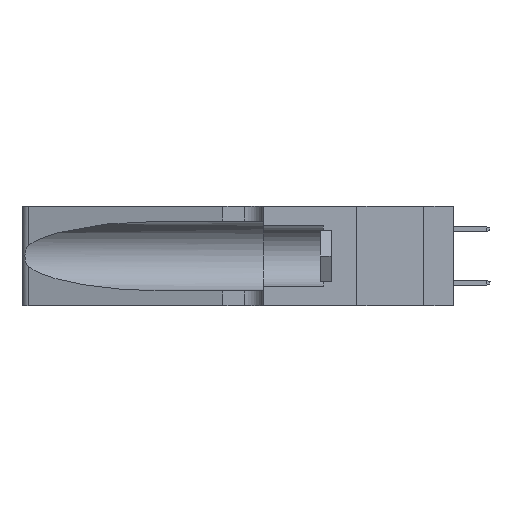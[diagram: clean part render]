
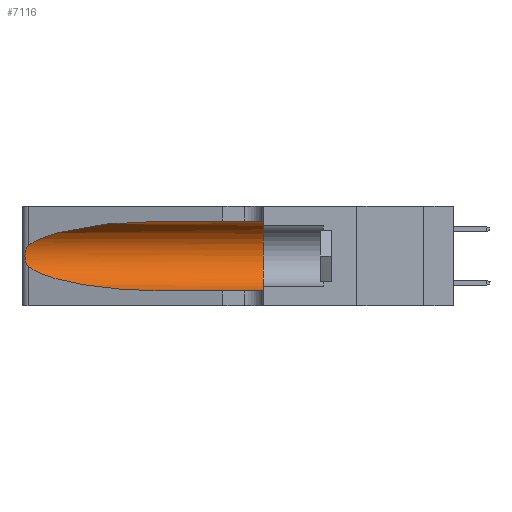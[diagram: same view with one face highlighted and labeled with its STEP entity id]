
A CAD part, left-side view. The second image highlights one B-rep face of the part: STEP entity #7116.
In plain terms, the highlighted cylindrical face has radius 3.308 mm (diameter 6.617 mm), a partial arc.
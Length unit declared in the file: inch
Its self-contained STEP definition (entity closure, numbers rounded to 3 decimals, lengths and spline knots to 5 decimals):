
#10 = CARTESIAN_POINT ( 'NONE',  ( 0.26075, 1.23896, 0.178 ) ) ;
#398 = CARTESIAN_POINT ( 'NONE',  ( 0.25487, 1.22718, 0.22369 ) ) ;
#905 = CARTESIAN_POINT ( 'NONE',  ( 0.18966, 0.96281, 0.31525 ) ) ;
#1256 = ORIENTED_EDGE ( 'NONE', *, *, #2125, .T. ) ;
#1506 = VERTEX_POINT ( 'NONE', #3675 ) ;
#1937 = EDGE_CURVE ( 'NONE', #20835, #1506, #25398, .T. ) ;
#2125 = EDGE_CURVE ( 'NONE', #20279, #20429, #20356, .T. ) ;
#3675 = CARTESIAN_POINT ( 'NONE',  ( 0.1305, 0.35, 0.31525 ) ) ;
#4053 = AXIS2_PLACEMENT_3D ( 'NONE', #25340, #15194, #23163 ) ;
#4141 = CARTESIAN_POINT ( 'NONE',  ( 0.25639, 1.23184, 0.21858 ) ) ;
#4383 = VECTOR ( 'NONE', #13588, 39.37008 ) ;
#4564 = ORIENTED_EDGE ( 'NONE', *, *, #13562, .T. ) ;
#5171 = CARTESIAN_POINT ( 'NONE',  ( 0.25487, 1.22718, 0.14631 ) ) ;
#5219 = EDGE_CURVE ( 'NONE', #1506, #20429, #9873, .T. ) ;
#6209 = CARTESIAN_POINT ( 'NONE',  ( 0.25487, 1.22718, 0.14631 ) ) ;
#6328 = AXIS2_PLACEMENT_3D ( 'NONE', #14900, #19466, #11002 ) ;
#6487 = CARTESIAN_POINT ( 'NONE',  ( 0.1305, 0.35, 0.05475 ) ) ;
#6963 = CARTESIAN_POINT ( 'NONE',  ( 0.2373, 1.15595, 0.08982 ) ) ;
#6987 = EDGE_LOOP ( 'NONE', ( #10252, #14027, #4564, #1256, #10451, #23169 ) ) ;
#7021 = FACE_OUTER_BOUND ( 'NONE', #6987, .T. ) ;
#7116 = ADVANCED_FACE ( 'NONE', ( #7021 ), #17094, .F. ) ;
#7597 = VERTEX_POINT ( 'NONE', #5171 ) ;
#7632 = CARTESIAN_POINT ( 'NONE',  ( 0.1305, 1.61858, 0.31525 ) ) ;
#7908 = CARTESIAN_POINT ( 'NONE',  ( 0.25487, 1.22718, 0.22369 ) ) ;
#8137 = CARTESIAN_POINT ( 'NONE',  ( 0.26018, 1.23835, 0.19895 ) ) ;
#8648 =( BOUNDED_CURVE ( )  B_SPLINE_CURVE ( 3, ( #18629, #905, #8768, #16670 ),
 .UNSPECIFIED., .F., .F. ) 
 B_SPLINE_CURVE_WITH_KNOTS ( ( 4, 4 ),
 ( 1.5708, 2.84003 ),
 .UNSPECIFIED. ) 
 CURVE ( )  GEOMETRIC_REPRESENTATION_ITEM ( )  RATIONAL_B_SPLINE_CURVE ( ( 1., 0.87, 0.87, 1. ) ) 
 REPRESENTATION_ITEM ( '' )  );
#8768 = CARTESIAN_POINT ( 'NONE',  ( 0.2373, 1.15595, 0.28018 ) ) ;
#9436 = EDGE_CURVE ( 'NONE', #20835, #11485, #8648, .T. ) ;
#9873 = CIRCLE ( 'NONE', #4053, 0.13025 ) ;
#10121 = B_SPLINE_CURVE_WITH_KNOTS ( 'NONE', 3,
 ( #398, #10203, #4141, #12021, #22041, #8137, #19950, #10, #16031, #17973, #14207, #23989, #22167, #6209 ),
 .UNSPECIFIED., .F., .F.,
 ( 4, 2, 2, 2, 2, 2, 4 ),
 ( 0., 0.00027, 0.00053, 0.00107, 0.0016, 0.00187, 0.00214 ),
 .UNSPECIFIED. ) ;
#10203 = CARTESIAN_POINT ( 'NONE',  ( 0.25555, 1.22994, 0.2215 ) ) ;
#10252 = ORIENTED_EDGE ( 'NONE', *, *, #9436, .T. ) ;
#10448 = CARTESIAN_POINT ( 'NONE',  ( 0.1305, 1.61858, 0.05475 ) ) ;
#10451 = ORIENTED_EDGE ( 'NONE', *, *, #5219, .F. ) ;
#11002 = DIRECTION ( 'NONE',  ( 0., 0., -1. ) ) ;
#11485 = VERTEX_POINT ( 'NONE', #7908 ) ;
#12021 = CARTESIAN_POINT ( 'NONE',  ( 0.25787, 1.23484, 0.2124 ) ) ;
#13562 = EDGE_CURVE ( 'NONE', #7597, #20279, #21255, .T. ) ;
#13588 = DIRECTION ( 'NONE',  ( 0., -1., 0. ) ) ;
#14027 = ORIENTED_EDGE ( 'NONE', *, *, #22087, .T. ) ;
#14207 = CARTESIAN_POINT ( 'NONE',  ( 0.25789, 1.23486, 0.15765 ) ) ;
#14439 = CARTESIAN_POINT ( 'NONE',  ( 0.1305, 0.72297, 0.31525 ) ) ;
#14900 = CARTESIAN_POINT ( 'NONE',  ( 0.1305, 1.61858, 0.185 ) ) ;
#15194 = DIRECTION ( 'NONE',  ( 0., 1., 0. ) ) ;
#16031 = CARTESIAN_POINT ( 'NONE',  ( 0.26017, 1.23833, 0.17102 ) ) ;
#16670 = CARTESIAN_POINT ( 'NONE',  ( 0.25487, 1.22718, 0.22369 ) ) ;
#17094 = CYLINDRICAL_SURFACE ( 'NONE', #6328, 0.13025 ) ;
#17973 = CARTESIAN_POINT ( 'NONE',  ( 0.25856, 1.23593, 0.16098 ) ) ;
#17991 = DIRECTION ( 'NONE',  ( 0., -1., 0. ) ) ;
#18629 = CARTESIAN_POINT ( 'NONE',  ( 0.1305, 0.72297, 0.31525 ) ) ;
#19466 = DIRECTION ( 'NONE',  ( 0., -1., 0. ) ) ;
#19575 = CARTESIAN_POINT ( 'NONE',  ( 0.1305, 0.72297, 0.05475 ) ) ;
#19950 = CARTESIAN_POINT ( 'NONE',  ( 0.26075, 1.23896, 0.19203 ) ) ;
#20279 = VERTEX_POINT ( 'NONE', #19575 ) ;
#20356 = LINE ( 'NONE', #10448, #21412 ) ;
#20429 = VERTEX_POINT ( 'NONE', #6487 ) ;
#20835 = VERTEX_POINT ( 'NONE', #14439 ) ;
#20973 = CARTESIAN_POINT ( 'NONE',  ( 0.1305, 0.72297, 0.05475 ) ) ;
#21255 =( BOUNDED_CURVE ( )  B_SPLINE_CURVE ( 3, ( #24729, #6963, #24854, #20973 ),
 .UNSPECIFIED., .F., .F. ) 
 B_SPLINE_CURVE_WITH_KNOTS ( ( 4, 4 ),
 ( 3.44316, 4.71239 ),
 .UNSPECIFIED. ) 
 CURVE ( )  GEOMETRIC_REPRESENTATION_ITEM ( )  RATIONAL_B_SPLINE_CURVE ( ( 1., 0.87, 0.87, 1. ) ) 
 REPRESENTATION_ITEM ( '' )  );
#21412 = VECTOR ( 'NONE', #17991, 39.37008 ) ;
#22041 = CARTESIAN_POINT ( 'NONE',  ( 0.25854, 1.2359, 0.20912 ) ) ;
#22087 = EDGE_CURVE ( 'NONE', #11485, #7597, #10121, .T. ) ;
#22167 = CARTESIAN_POINT ( 'NONE',  ( 0.25555, 1.22993, 0.14849 ) ) ;
#23163 = DIRECTION ( 'NONE',  ( 0., 0., 1. ) ) ;
#23169 = ORIENTED_EDGE ( 'NONE', *, *, #1937, .F. ) ;
#23989 = CARTESIAN_POINT ( 'NONE',  ( 0.25639, 1.23186, 0.15144 ) ) ;
#24729 = CARTESIAN_POINT ( 'NONE',  ( 0.25487, 1.22718, 0.14631 ) ) ;
#24854 = CARTESIAN_POINT ( 'NONE',  ( 0.18966, 0.96281, 0.05475 ) ) ;
#25340 = CARTESIAN_POINT ( 'NONE',  ( 0.1305, 0.35, 0.185 ) ) ;
#25398 = LINE ( 'NONE', #7632, #4383 ) ;
